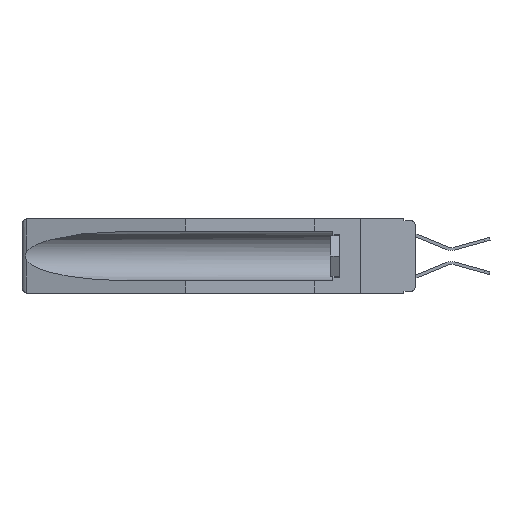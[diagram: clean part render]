
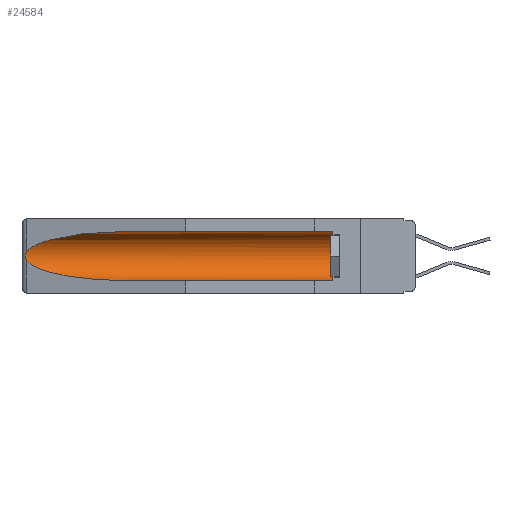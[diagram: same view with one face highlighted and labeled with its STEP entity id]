
A CAD part, left-side view. The second image highlights one B-rep face of the part: STEP entity #24584.
In plain terms, the highlighted cylindrical face has radius 2.857 mm (diameter 5.715 mm), a partial arc.
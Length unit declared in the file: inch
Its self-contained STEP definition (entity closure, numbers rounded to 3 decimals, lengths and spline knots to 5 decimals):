
#1082 = VERTEX_POINT ( 'NONE', #16443 ) ;
#1721 = CARTESIAN_POINT ( 'NONE',  ( 0.26654, 1.53092, -0.15636 ) ) ;
#2003 = CARTESIAN_POINT ( 'NONE',  ( 0.26537, 1.52718, -0.19328 ) ) ;
#2085 = ORIENTED_EDGE ( 'NONE', *, *, #8873, .T. ) ;
#2287 = CARTESIAN_POINT ( 'NONE',  ( 0.155, -0.30754, -0.059 ) ) ;
#2307 = CARTESIAN_POINT ( 'NONE',  ( 0.155, 0.126, -0.1715 ) ) ;
#2968 = DIRECTION ( 'NONE',  ( 0., 1., 0. ) ) ;
#3148 = CARTESIAN_POINT ( 'NONE',  ( 0.25451, 1.48313, -0.24835 ) ) ;
#4185 = CARTESIAN_POINT ( 'NONE',  ( 0.26655, 1.53094, -0.18657 ) ) ;
#4365 =( BOUNDED_CURVE ( )  B_SPLINE_CURVE ( 3, ( #20044, #7284, #11684, #9275 ),
 .UNSPECIFIED., .F., .F. ) 
 B_SPLINE_CURVE_WITH_KNOTS ( ( 4, 4 ),
 ( 4.71239, 6.08839 ),
 .UNSPECIFIED. ) 
 CURVE ( )  GEOMETRIC_REPRESENTATION_ITEM ( )  RATIONAL_B_SPLINE_CURVE ( ( 1., 0.848, 0.848, 1. ) ) 
 REPRESENTATION_ITEM ( '' )  );
#4745 = EDGE_CURVE ( 'NONE', #17187, #12940, #4365, .T. ) ;
#5039 = CARTESIAN_POINT ( 'NONE',  ( 0.155, -0.30754, -0.284 ) ) ;
#5306 = CARTESIAN_POINT ( 'NONE',  ( 0.21114, 1.30732, -0.284 ) ) ;
#6280 = CIRCLE ( 'NONE', #7819, 0.1125 ) ;
#6316 = CARTESIAN_POINT ( 'NONE',  ( 0.2673, 1.53269, -0.17917 ) ) ;
#6412 = CARTESIAN_POINT ( 'NONE',  ( 0.2675, 1.53308, -0.17534 ) ) ;
#6596 = ORIENTED_EDGE ( 'NONE', *, *, #24454, .T. ) ;
#6921 = FACE_OUTER_BOUND ( 'NONE', #26341, .T. ) ;
#6956 = DIRECTION ( 'NONE',  ( 0., 1., 0. ) ) ;
#7284 = CARTESIAN_POINT ( 'NONE',  ( 0.21114, 1.30732, -0.059 ) ) ;
#7729 = CARTESIAN_POINT ( 'NONE',  ( 0.26537, 1.52718, -0.14972 ) ) ;
#7819 = AXIS2_PLACEMENT_3D ( 'NONE', #2307, #8775, #17226 ) ;
#7994 = CARTESIAN_POINT ( 'NONE',  ( 0.155, 1.07973, -0.284 ) ) ;
#8775 = DIRECTION ( 'NONE',  ( 0., -1., 0. ) ) ;
#8873 = EDGE_CURVE ( 'NONE', #26029, #10963, #20486, .T. ) ;
#9270 = CYLINDRICAL_SURFACE ( 'NONE', #22908, 0.1125 ) ;
#9275 = CARTESIAN_POINT ( 'NONE',  ( 0.26537, 1.52718, -0.14972 ) ) ;
#9310 = VECTOR ( 'NONE', #2968, 39.37008 ) ;
#9479 = CARTESIAN_POINT ( 'NONE',  ( 0.26537, 1.52718, -0.14972 ) ) ;
#10963 = VERTEX_POINT ( 'NONE', #7994 ) ;
#11684 = CARTESIAN_POINT ( 'NONE',  ( 0.25451, 1.48313, -0.09465 ) ) ;
#11749 = EDGE_CURVE ( 'NONE', #1082, #10963, #23387, .T. ) ;
#12491 = CARTESIAN_POINT ( 'NONE',  ( 0.2673, 1.5327, -0.16383 ) ) ;
#12940 = VERTEX_POINT ( 'NONE', #9479 ) ;
#13604 = ORIENTED_EDGE ( 'NONE', *, *, #16269, .T. ) ;
#15131 = DIRECTION ( 'NONE',  ( 0., 0., 1. ) ) ;
#15978 = VERTEX_POINT ( 'NONE', #27142 ) ;
#16227 = LINE ( 'NONE', #2287, #19584 ) ;
#16269 = EDGE_CURVE ( 'NONE', #15978, #17187, #16227, .T. ) ;
#16374 = CARTESIAN_POINT ( 'NONE',  ( 0.26597, 1.52961, -0.15275 ) ) ;
#16443 = CARTESIAN_POINT ( 'NONE',  ( 0.155, 0.126, -0.284 ) ) ;
#16590 = CARTESIAN_POINT ( 'NONE',  ( 0.155, 1.07973, -0.059 ) ) ;
#16740 = CARTESIAN_POINT ( 'NONE',  ( 0.2675, 1.53308, -0.16763 ) ) ;
#17187 = VERTEX_POINT ( 'NONE', #16590 ) ;
#17226 = DIRECTION ( 'NONE',  ( 0., 0., 1. ) ) ;
#17229 = ORIENTED_EDGE ( 'NONE', *, *, #4745, .T. ) ;
#18232 = CARTESIAN_POINT ( 'NONE',  ( 0.26537, 1.52718, -0.19328 ) ) ;
#18333 = CARTESIAN_POINT ( 'NONE',  ( 0.155, 1.07973, -0.284 ) ) ;
#18971 = ORIENTED_EDGE ( 'NONE', *, *, #11749, .F. ) ;
#19584 = VECTOR ( 'NONE', #6956, 39.37008 ) ;
#20044 = CARTESIAN_POINT ( 'NONE',  ( 0.155, 1.07973, -0.059 ) ) ;
#20486 =( BOUNDED_CURVE ( )  B_SPLINE_CURVE ( 3, ( #18232, #3148, #5306, #18333 ),
 .UNSPECIFIED., .F., .F. ) 
 B_SPLINE_CURVE_WITH_KNOTS ( ( 4, 4 ),
 ( 0.1948, 1.5708 ),
 .UNSPECIFIED. ) 
 CURVE ( )  GEOMETRIC_REPRESENTATION_ITEM ( )  RATIONAL_B_SPLINE_CURVE ( ( 1., 0.848, 0.848, 1. ) ) 
 REPRESENTATION_ITEM ( '' )  );
#21475 = DIRECTION ( 'NONE',  ( 0., 1., 0. ) ) ;
#21867 = CARTESIAN_POINT ( 'NONE',  ( 0.26537, 1.52718, -0.19328 ) ) ;
#22908 = AXIS2_PLACEMENT_3D ( 'NONE', #25829, #21475, #15131 ) ;
#23387 = LINE ( 'NONE', #5039, #9310 ) ;
#23634 = ORIENTED_EDGE ( 'NONE', *, *, #24049, .T. ) ;
#24049 = EDGE_CURVE ( 'NONE', #1082, #15978, #6280, .T. ) ;
#24454 = EDGE_CURVE ( 'NONE', #12940, #26029, #25080, .T. ) ;
#24584 = ADVANCED_FACE ( 'NONE', ( #6921 ), #9270, .F. ) ;
#25080 = B_SPLINE_CURVE_WITH_KNOTS ( 'NONE', 3,
 ( #7729, #16374, #1721, #12491, #16740, #6412, #6316, #4185, #27418, #2003 ),
 .UNSPECIFIED., .F., .F.,
 ( 4, 2, 2, 2, 4 ),
 ( 0., 0.00029, 0.00058, 0.00087, 0.00117 ),
 .UNSPECIFIED. ) ;
#25829 = CARTESIAN_POINT ( 'NONE',  ( 0.155, -0.30754, -0.1715 ) ) ;
#26029 = VERTEX_POINT ( 'NONE', #21867 ) ;
#26341 = EDGE_LOOP ( 'NONE', ( #17229, #6596, #2085, #18971, #23634, #13604 ) ) ;
#27142 = CARTESIAN_POINT ( 'NONE',  ( 0.155, 0.126, -0.059 ) ) ;
#27418 = CARTESIAN_POINT ( 'NONE',  ( 0.26597, 1.5296, -0.19026 ) ) ;
